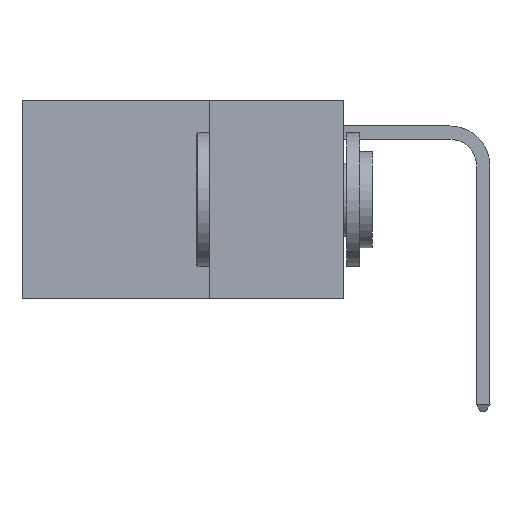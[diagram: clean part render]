
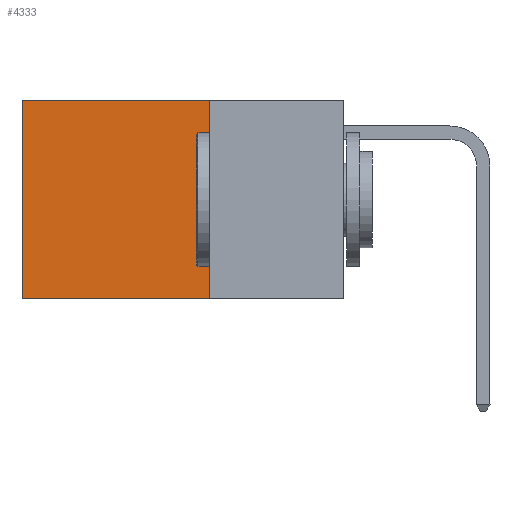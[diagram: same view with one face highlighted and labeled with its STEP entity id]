
A CAD part, left-side view. The second image highlights one B-rep face of the part: STEP entity #4333.
In plain terms, the highlighted planar face has unit normal (-1, 0, 0).
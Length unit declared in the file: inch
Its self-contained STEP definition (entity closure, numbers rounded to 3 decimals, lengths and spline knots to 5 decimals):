
#550 = ORIENTED_EDGE ( 'NONE', *, *, #8762, .F. ) ;
#587 = DIRECTION ( 'NONE',  ( 0., 0., -1. ) ) ;
#634 = CARTESIAN_POINT ( 'NONE',  ( 0.2625, 0.25, 0. ) ) ;
#834 = VERTEX_POINT ( 'NONE', #4459 ) ;
#1467 = ORIENTED_EDGE ( 'NONE', *, *, #7809, .F. ) ;
#1589 = CARTESIAN_POINT ( 'NONE',  ( 0.2625, 0.25, -0.37 ) ) ;
#1985 = EDGE_CURVE ( 'NONE', #5522, #834, #5461, .T. ) ;
#2014 = VERTEX_POINT ( 'NONE', #8250 ) ;
#2155 = CARTESIAN_POINT ( 'NONE',  ( 0.2625, 0.25, 0. ) ) ;
#3318 = CARTESIAN_POINT ( 'NONE',  ( 0.2625, 0.25, -0.37 ) ) ;
#4089 = DIRECTION ( 'NONE',  ( 1., 0., 0. ) ) ;
#4333 = ADVANCED_FACE ( 'NONE', ( #7574 ), #8922, .F. ) ;
#4388 = DIRECTION ( 'NONE',  ( 0., 0., -1. ) ) ;
#4459 = CARTESIAN_POINT ( 'NONE',  ( 0.2625, 0.6, 0. ) ) ;
#4706 = DIRECTION ( 'NONE',  ( 0., 1., 0. ) ) ;
#4756 = DIRECTION ( 'NONE',  ( 0., 0., -1. ) ) ;
#4854 = VERTEX_POINT ( 'NONE', #1589 ) ;
#5461 = LINE ( 'NONE', #634, #8151 ) ;
#5499 = VECTOR ( 'NONE', #9026, 39.37008 ) ;
#5522 = VERTEX_POINT ( 'NONE', #6878 ) ;
#5676 = ORIENTED_EDGE ( 'NONE', *, *, #7161, .T. ) ;
#5834 = CARTESIAN_POINT ( 'NONE',  ( 0.2625, 0.25, 0. ) ) ;
#5976 = AXIS2_PLACEMENT_3D ( 'NONE', #2155, #4089, #587 ) ;
#6112 = VECTOR ( 'NONE', #4756, 39.37008 ) ;
#6870 = LINE ( 'NONE', #3318, #5499 ) ;
#6878 = CARTESIAN_POINT ( 'NONE',  ( 0.2625, 0.25, 0. ) ) ;
#7161 = EDGE_CURVE ( 'NONE', #834, #2014, #8286, .T. ) ;
#7240 = VECTOR ( 'NONE', #4388, 39.37008 ) ;
#7574 = FACE_OUTER_BOUND ( 'NONE', #7803, .T. ) ;
#7803 = EDGE_LOOP ( 'NONE', ( #5676, #550, #1467, #8726 ) ) ;
#7809 = EDGE_CURVE ( 'NONE', #5522, #4854, #8057, .T. ) ;
#8057 = LINE ( 'NONE', #5834, #7240 ) ;
#8151 = VECTOR ( 'NONE', #4706, 39.37008 ) ;
#8250 = CARTESIAN_POINT ( 'NONE',  ( 0.2625, 0.6, -0.37 ) ) ;
#8286 = LINE ( 'NONE', #8333, #6112 ) ;
#8333 = CARTESIAN_POINT ( 'NONE',  ( 0.2625, 0.6, 0. ) ) ;
#8726 = ORIENTED_EDGE ( 'NONE', *, *, #1985, .T. ) ;
#8762 = EDGE_CURVE ( 'NONE', #4854, #2014, #6870, .T. ) ;
#8922 = PLANE ( 'NONE',  #5976 ) ;
#9026 = DIRECTION ( 'NONE',  ( 0., 1., 0. ) ) ;
